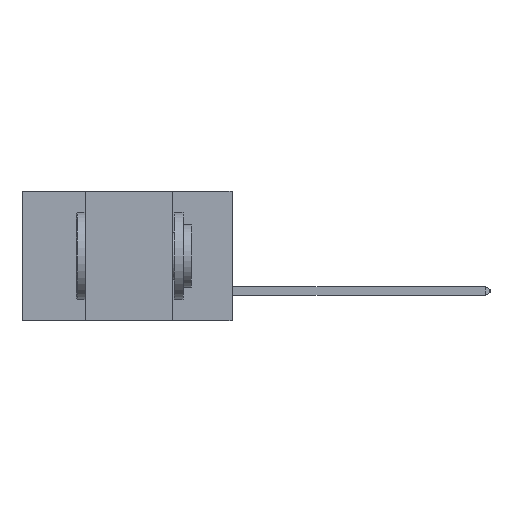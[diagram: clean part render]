
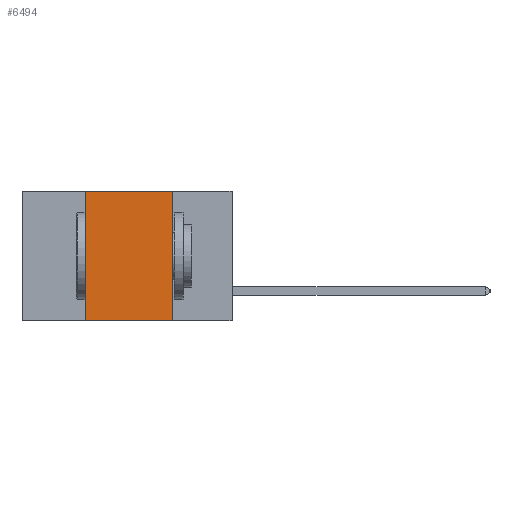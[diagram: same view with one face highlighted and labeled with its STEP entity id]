
A CAD part, left-side view. The second image highlights one B-rep face of the part: STEP entity #6494.
In plain terms, the highlighted planar face has unit normal (-1, 0, 0).
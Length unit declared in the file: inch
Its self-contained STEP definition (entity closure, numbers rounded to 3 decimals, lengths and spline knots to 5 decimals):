
#1001 = VERTEX_POINT ( 'NONE', #13590 ) ;
#3052 = VECTOR ( 'NONE', #4989, 39.37008 ) ;
#3236 = VERTEX_POINT ( 'NONE', #14537 ) ;
#3771 = VECTOR ( 'NONE', #6008, 39.37008 ) ;
#4301 = AXIS2_PLACEMENT_3D ( 'NONE', #13824, #15123, #7150 ) ;
#4444 = PLANE ( 'NONE',  #4301 ) ;
#4989 = DIRECTION ( 'NONE',  ( 0., 0., 1. ) ) ;
#5526 = CARTESIAN_POINT ( 'NONE',  ( 0., 0.6, -0.37 ) ) ;
#6008 = DIRECTION ( 'NONE',  ( 0., -1., 0. ) ) ;
#6121 = EDGE_CURVE ( 'NONE', #1001, #14353, #14150, .T. ) ;
#6494 = ADVANCED_FACE ( 'NONE', ( #11417 ), #4444, .F. ) ;
#6690 = LINE ( 'NONE', #14364, #3052 ) ;
#7008 = CARTESIAN_POINT ( 'NONE',  ( 0., 0.17, -0.37 ) ) ;
#7096 = ORIENTED_EDGE ( 'NONE', *, *, #7867, .F. ) ;
#7150 = DIRECTION ( 'NONE',  ( 0., 0., -1. ) ) ;
#7162 = CARTESIAN_POINT ( 'NONE',  ( 0., 0.42, 0. ) ) ;
#7439 = LINE ( 'NONE', #5526, #17563 ) ;
#7867 = EDGE_CURVE ( 'NONE', #14986, #1001, #10913, .T. ) ;
#8678 = CARTESIAN_POINT ( 'NONE',  ( 0., 0.6, 0. ) ) ;
#8978 = DIRECTION ( 'NONE',  ( 0., 0., -1. ) ) ;
#9553 = DIRECTION ( 'NONE',  ( 0., -1., 0. ) ) ;
#9825 = ORIENTED_EDGE ( 'NONE', *, *, #6121, .F. ) ;
#10668 = ORIENTED_EDGE ( 'NONE', *, *, #17008, .F. ) ;
#10913 = LINE ( 'NONE', #8678, #3771 ) ;
#11417 = FACE_OUTER_BOUND ( 'NONE', #14419, .T. ) ;
#13590 = CARTESIAN_POINT ( 'NONE',  ( 0., 0.17, 0. ) ) ;
#13650 = EDGE_CURVE ( 'NONE', #3236, #14353, #7439, .T. ) ;
#13824 = CARTESIAN_POINT ( 'NONE',  ( 0., 0.6, 0. ) ) ;
#14150 = LINE ( 'NONE', #15660, #16776 ) ;
#14353 = VERTEX_POINT ( 'NONE', #7008 ) ;
#14364 = CARTESIAN_POINT ( 'NONE',  ( 0., 0.42, 0. ) ) ;
#14419 = EDGE_LOOP ( 'NONE', ( #9825, #7096, #10668, #14634 ) ) ;
#14537 = CARTESIAN_POINT ( 'NONE',  ( 0., 0.42, -0.37 ) ) ;
#14634 = ORIENTED_EDGE ( 'NONE', *, *, #13650, .T. ) ;
#14986 = VERTEX_POINT ( 'NONE', #7162 ) ;
#15123 = DIRECTION ( 'NONE',  ( 1., 0., 0. ) ) ;
#15660 = CARTESIAN_POINT ( 'NONE',  ( 0., 0.17, 0. ) ) ;
#16776 = VECTOR ( 'NONE', #8978, 39.37008 ) ;
#17008 = EDGE_CURVE ( 'NONE', #3236, #14986, #6690, .T. ) ;
#17563 = VECTOR ( 'NONE', #9553, 39.37008 ) ;
